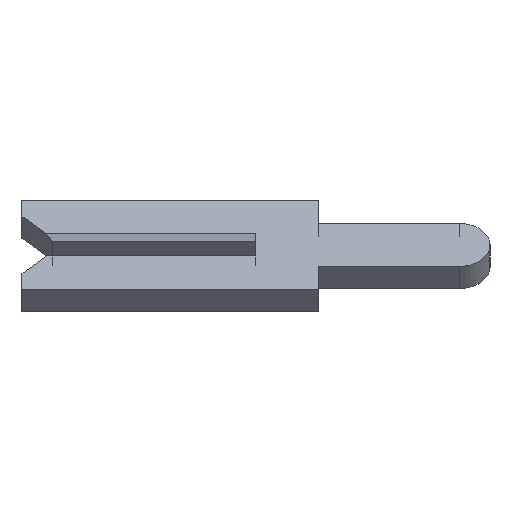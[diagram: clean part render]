
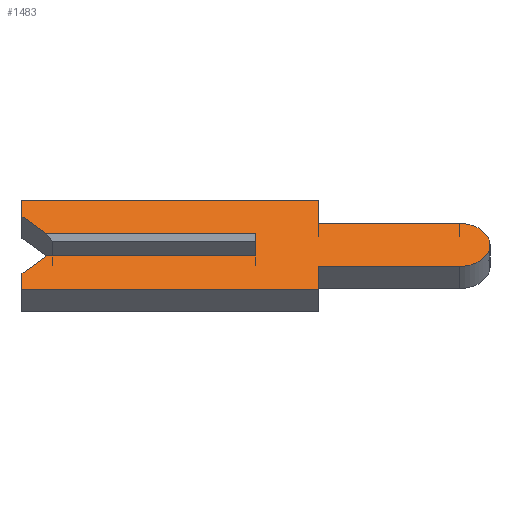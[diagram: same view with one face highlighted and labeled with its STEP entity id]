
A CAD part, left-side view. The second image highlights one B-rep face of the part: STEP entity #1483.
In plain terms, the highlighted face is planar.
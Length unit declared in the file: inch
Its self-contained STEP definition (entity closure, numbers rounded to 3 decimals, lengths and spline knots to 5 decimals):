
#42 = VECTOR ( 'NONE', #376, 39.37008 ) ;
#65 = EDGE_CURVE ( 'NONE', #2107, #800, #1016, .T. ) ;
#74 = LINE ( 'NONE', #1891, #876 ) ;
#77 = LINE ( 'NONE', #1554, #1336 ) ;
#103 = LINE ( 'NONE', #1569, #420 ) ;
#179 = DIRECTION ( 'NONE',  ( 0., -1., 0. ) ) ;
#184 = DIRECTION ( 'NONE',  ( 0., 0., 1. ) ) ;
#185 = AXIS2_PLACEMENT_3D ( 'NONE', #1365, #1694, #2025 ) ;
#212 = DIRECTION ( 'NONE',  ( 0., 0., 1. ) ) ;
#230 = CARTESIAN_POINT ( 'NONE',  ( -0.01, 0.15, -0.026 ) ) ;
#258 = ORIENTED_EDGE ( 'NONE', *, *, #482, .F. ) ;
#284 = ORIENTED_EDGE ( 'NONE', *, *, #65, .F. ) ;
#309 = AXIS2_PLACEMENT_3D ( 'NONE', #1317, #1320, #998 ) ;
#313 = ORIENTED_EDGE ( 'NONE', *, *, #1183, .F. ) ;
#314 = CARTESIAN_POINT ( 'NONE',  ( -0.01, -0.04, 0.04 ) ) ;
#333 = ORIENTED_EDGE ( 'NONE', *, *, #1197, .F. ) ;
#337 = ORIENTED_EDGE ( 'NONE', *, *, #757, .F. ) ;
#343 = ORIENTED_EDGE ( 'NONE', *, *, #1782, .F. ) ;
#376 = DIRECTION ( 'NONE',  ( 0., 0., -1. ) ) ;
#383 = CARTESIAN_POINT ( 'NONE',  ( -0.01, -0.04, 0.0195 ) ) ;
#392 = CARTESIAN_POINT ( 'NONE',  ( -0.01, -0.04, -0.0195 ) ) ;
#398 = ORIENTED_EDGE ( 'NONE', *, *, #1343, .T. ) ;
#420 = VECTOR ( 'NONE', #1743, 39.37008 ) ;
#456 = EDGE_CURVE ( 'NONE', #1859, #2107, #74, .T. ) ;
#476 = ORIENTED_EDGE ( 'NONE', *, *, #660, .F. ) ;
#478 = ORIENTED_EDGE ( 'NONE', *, *, #501, .F. ) ;
#482 = EDGE_CURVE ( 'NONE', #1760, #1620, #627, .T. ) ;
#501 = EDGE_CURVE ( 'NONE', #1282, #1600, #2021, .T. ) ;
#520 = ORIENTED_EDGE ( 'NONE', *, *, #1133, .F. ) ;
#563 = DIRECTION ( 'NONE',  ( 0., 1., 0. ) ) ;
#617 = VECTOR ( 'NONE', #563, 39.37008 ) ;
#627 = LINE ( 'NONE', #1234, #910 ) ;
#648 = CARTESIAN_POINT ( 'NONE',  ( -0.01, 0., -0.01 ) ) ;
#660 = EDGE_CURVE ( 'NONE', #1762, #852, #668, .T. ) ;
#668 = LINE ( 'NONE', #896, #1025 ) ;
#686 = CARTESIAN_POINT ( 'NONE',  ( -0.01, -0.04, 0.04 ) ) ;
#696 = DIRECTION ( 'NONE',  ( 0., 0.707, 0.707 ) ) ;
#697 = EDGE_LOOP ( 'NONE', ( #398, #313, #258, #1138, #476, #1022, #478, #333, #966, #520, #284, #1893, #337, #343 ) ) ;
#703 = DIRECTION ( 'NONE',  ( 0., -1., 0. ) ) ;
#704 = EDGE_CURVE ( 'NONE', #1600, #1762, #77, .T. ) ;
#709 = DIRECTION ( 'NONE',  ( 0., 1., 0. ) ) ;
#737 = CARTESIAN_POINT ( 'NONE',  ( -0.01, -0.04, -0.0195 ) ) ;
#753 = CARTESIAN_POINT ( 'NONE',  ( -0.01, -0.04, 0.0195 ) ) ;
#757 = EDGE_CURVE ( 'NONE', #1264, #1859, #103, .T. ) ;
#800 = VERTEX_POINT ( 'NONE', #753 ) ;
#835 = DIRECTION ( 'NONE',  ( 0., -0.707, 0.707 ) ) ;
#852 = VERTEX_POINT ( 'NONE', #230 ) ;
#876 = VECTOR ( 'NONE', #179, 39.37008 ) ;
#893 = LINE ( 'NONE', #1529, #1658 ) ;
#896 = CARTESIAN_POINT ( 'NONE',  ( -0.01, 0.15, -0.026 ) ) ;
#910 = VECTOR ( 'NONE', #703, 39.37008 ) ;
#966 = ORIENTED_EDGE ( 'NONE', *, *, #1939, .F. ) ;
#979 = DIRECTION ( 'NONE',  ( 0., -1., 0. ) ) ;
#990 = CARTESIAN_POINT ( 'NONE',  ( -0.01, -0.1305, -0.0195 ) ) ;
#998 = DIRECTION ( 'NONE',  ( 0., 0., -1. ) ) ;
#1016 = LINE ( 'NONE', #314, #1204 ) ;
#1022 = ORIENTED_EDGE ( 'NONE', *, *, #704, .F. ) ;
#1025 = VECTOR ( 'NONE', #184, 39.37008 ) ;
#1028 = CARTESIAN_POINT ( 'NONE',  ( -0.01, 0.15, 0.04 ) ) ;
#1087 = FACE_OUTER_BOUND ( 'NONE', #697, .T. ) ;
#1116 = VECTOR ( 'NONE', #979, 39.37008 ) ;
#1133 = EDGE_CURVE ( 'NONE', #800, #1230, #1623, .T. ) ;
#1138 = ORIENTED_EDGE ( 'NONE', *, *, #1915, .F. ) ;
#1183 = EDGE_CURVE ( 'NONE', #1620, #1402, #1546, .T. ) ;
#1197 = EDGE_CURVE ( 'NONE', #1406, #1282, #1244, .T. ) ;
#1204 = VECTOR ( 'NONE', #1499, 39.37008 ) ;
#1230 = VERTEX_POINT ( 'NONE', #1771 ) ;
#1234 = CARTESIAN_POINT ( 'NONE',  ( -0.01, -0.1305, -0.01 ) ) ;
#1244 = LINE ( 'NONE', #392, #617 ) ;
#1247 = VECTOR ( 'NONE', #696, 39.37008 ) ;
#1255 = CARTESIAN_POINT ( 'NONE',  ( -0.01, 0., 0.0065 ) ) ;
#1264 = VERTEX_POINT ( 'NONE', #1409 ) ;
#1272 = VECTOR ( 'NONE', #1574, 39.37008 ) ;
#1282 = VERTEX_POINT ( 'NONE', #737 ) ;
#1317 = CARTESIAN_POINT ( 'NONE',  ( -0.01, -0.1305, 0. ) ) ;
#1320 = DIRECTION ( 'NONE',  ( 1., 0., 0. ) ) ;
#1335 = CARTESIAN_POINT ( 'NONE',  ( -0.01, 0., 0.01 ) ) ;
#1336 = VECTOR ( 'NONE', #709, 39.37008 ) ;
#1343 = EDGE_CURVE ( 'NONE', #1516, #1402, #1524, .T. ) ;
#1360 = CARTESIAN_POINT ( 'NONE',  ( -0.01, 0.15, -0.04 ) ) ;
#1365 = CARTESIAN_POINT ( 'NONE',  ( -0.01, -0.1305, 0. ) ) ;
#1375 = CARTESIAN_POINT ( 'NONE',  ( -0.01, -0.04, -0.04 ) ) ;
#1402 = VERTEX_POINT ( 'NONE', #1335 ) ;
#1406 = VERTEX_POINT ( 'NONE', #990 ) ;
#1409 = CARTESIAN_POINT ( 'NONE',  ( -0.01, 0.15, 0.026 ) ) ;
#1483 = ADVANCED_FACE ( 'NONE', ( #1087 ), #2000, .F. ) ;
#1488 = CARTESIAN_POINT ( 'NONE',  ( -0.01, 0.134, -0.01 ) ) ;
#1498 = CARTESIAN_POINT ( 'NONE',  ( -0.01, -0.04, -0.04 ) ) ;
#1499 = DIRECTION ( 'NONE',  ( 0., 0., -1. ) ) ;
#1516 = VERTEX_POINT ( 'NONE', #2162 ) ;
#1524 = LINE ( 'NONE', #1834, #1116 ) ;
#1529 = CARTESIAN_POINT ( 'NONE',  ( -0.01, 0.1305, -0.0065 ) ) ;
#1546 = LINE ( 'NONE', #1255, #1710 ) ;
#1554 = CARTESIAN_POINT ( 'NONE',  ( -0.01, 0.15, -0.04 ) ) ;
#1569 = CARTESIAN_POINT ( 'NONE',  ( -0.01, 0.15, 0.026 ) ) ;
#1574 = DIRECTION ( 'NONE',  ( 0., -1., 0. ) ) ;
#1600 = VERTEX_POINT ( 'NONE', #1498 ) ;
#1606 = CIRCLE ( 'NONE', #185, 0.0195 ) ;
#1620 = VERTEX_POINT ( 'NONE', #648 ) ;
#1623 = LINE ( 'NONE', #383, #1272 ) ;
#1658 = VECTOR ( 'NONE', #835, 39.37008 ) ;
#1694 = DIRECTION ( 'NONE',  ( 1., 0., 0. ) ) ;
#1710 = VECTOR ( 'NONE', #212, 39.37008 ) ;
#1743 = DIRECTION ( 'NONE',  ( 0., 0., 1. ) ) ;
#1760 = VERTEX_POINT ( 'NONE', #1488 ) ;
#1762 = VERTEX_POINT ( 'NONE', #1360 ) ;
#1771 = CARTESIAN_POINT ( 'NONE',  ( -0.01, -0.1305, 0.0195 ) ) ;
#1782 = EDGE_CURVE ( 'NONE', #1516, #1264, #2061, .T. ) ;
#1834 = CARTESIAN_POINT ( 'NONE',  ( -0.01, 0.15, 0.01 ) ) ;
#1859 = VERTEX_POINT ( 'NONE', #1028 ) ;
#1891 = CARTESIAN_POINT ( 'NONE',  ( -0.01, 0.15, 0.04 ) ) ;
#1893 = ORIENTED_EDGE ( 'NONE', *, *, #456, .F. ) ;
#1915 = EDGE_CURVE ( 'NONE', #852, #1760, #893, .T. ) ;
#1939 = EDGE_CURVE ( 'NONE', #1230, #1406, #1606, .T. ) ;
#2000 = PLANE ( 'NONE',  #309 ) ;
#2021 = LINE ( 'NONE', #1375, #42 ) ;
#2025 = DIRECTION ( 'NONE',  ( 0., 0., -1. ) ) ;
#2049 = CARTESIAN_POINT ( 'NONE',  ( -0.01, 0.1305, 0.0065 ) ) ;
#2061 = LINE ( 'NONE', #2049, #1247 ) ;
#2107 = VERTEX_POINT ( 'NONE', #686 ) ;
#2162 = CARTESIAN_POINT ( 'NONE',  ( -0.01, 0.134, 0.01 ) ) ;
